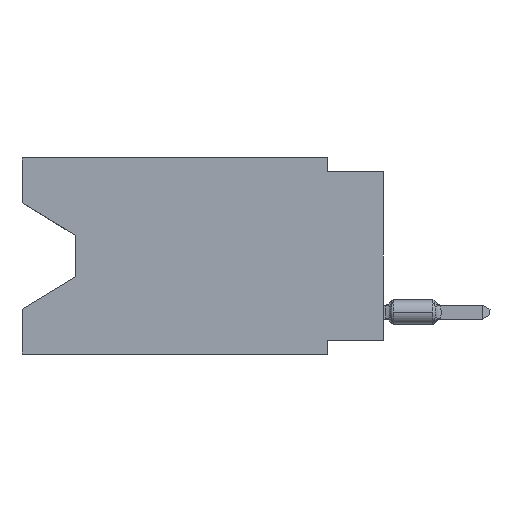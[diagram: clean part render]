
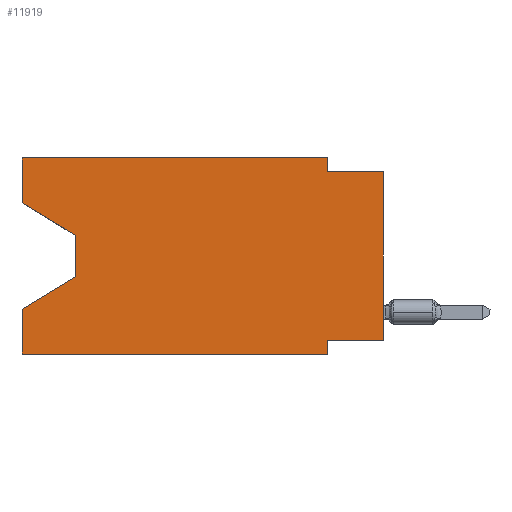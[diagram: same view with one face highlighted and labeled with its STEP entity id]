
A CAD part, left-side view. The second image highlights one B-rep face of the part: STEP entity #11919.
In plain terms, the highlighted planar face has unit normal (-1, 0, 0).
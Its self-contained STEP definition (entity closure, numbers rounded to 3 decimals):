
#265 = DIRECTION ( 'NONE',  ( 0., 0., 1. ) ) ;
#654 = ORIENTED_EDGE ( 'NONE', *, *, #4400, .F. ) ;
#823 = PLANE ( 'NONE',  #14181 ) ;
#1098 = EDGE_CURVE ( 'NONE', #6949, #5626, #3951, .T. ) ;
#1354 = CARTESIAN_POINT ( 'NONE',  ( 0., 2.54, -8.89 ) ) ;
#1677 = VERTEX_POINT ( 'NONE', #11141 ) ;
#1715 = VERTEX_POINT ( 'NONE', #12490 ) ;
#1744 = CARTESIAN_POINT ( 'NONE',  ( 0., 2.54, -8.255 ) ) ;
#1812 = ORIENTED_EDGE ( 'NONE', *, *, #13902, .F. ) ;
#1820 = DIRECTION ( 'NONE',  ( 0., 0., -1. ) ) ;
#2035 = CARTESIAN_POINT ( 'NONE',  ( 0., 16.383, 0. ) ) ;
#2098 = VECTOR ( 'NONE', #13037, 1000. ) ;
#2214 = VERTEX_POINT ( 'NONE', #4270 ) ;
#2402 = CARTESIAN_POINT ( 'NONE',  ( 0., 16.383, -8.89 ) ) ;
#2649 = CARTESIAN_POINT ( 'NONE',  ( 0., 13.97, -5.385 ) ) ;
#2692 = EDGE_CURVE ( 'NONE', #5484, #7489, #3575, .T. ) ;
#2698 = DIRECTION ( 'NONE',  ( 0., -1., 0. ) ) ;
#2728 = DIRECTION ( 'NONE',  ( 0., 0., -1. ) ) ;
#2739 = VERTEX_POINT ( 'NONE', #2649 ) ;
#2799 = EDGE_CURVE ( 'NONE', #1677, #6949, #7518, .T. ) ;
#2878 = ORIENTED_EDGE ( 'NONE', *, *, #2692, .F. ) ;
#2987 = CARTESIAN_POINT ( 'NONE',  ( 0., 0., -0.635 ) ) ;
#3268 = EDGE_CURVE ( 'NONE', #1715, #4939, #3776, .T. ) ;
#3575 = LINE ( 'NONE', #5774, #4999 ) ;
#3587 = VECTOR ( 'NONE', #6198, 1000. ) ;
#3776 = LINE ( 'NONE', #8427, #2098 ) ;
#3791 = VECTOR ( 'NONE', #4378, 1000. ) ;
#3951 = LINE ( 'NONE', #10875, #9055 ) ;
#3972 = LINE ( 'NONE', #7248, #12291 ) ;
#4261 = VERTEX_POINT ( 'NONE', #2402 ) ;
#4266 = VECTOR ( 'NONE', #12143, 1000. ) ;
#4270 = CARTESIAN_POINT ( 'NONE',  ( 0., 13.97, -3.505 ) ) ;
#4378 = DIRECTION ( 'NONE',  ( 0., 0.855, -0.519 ) ) ;
#4400 = EDGE_CURVE ( 'NONE', #4261, #10344, #7506, .T. ) ;
#4460 = EDGE_CURVE ( 'NONE', #4261, #5626, #14266, .T. ) ;
#4526 = CARTESIAN_POINT ( 'NONE',  ( 0., 0., 0. ) ) ;
#4890 = DIRECTION ( 'NONE',  ( 0., 0., 1. ) ) ;
#4939 = VERTEX_POINT ( 'NONE', #2987 ) ;
#4984 = LINE ( 'NONE', #10981, #3587 ) ;
#4999 = VECTOR ( 'NONE', #8222, 1000. ) ;
#5248 = EDGE_CURVE ( 'NONE', #2214, #2739, #11901, .T. ) ;
#5326 = EDGE_LOOP ( 'NONE', ( #6303, #9908, #8295, #654, #8242, #13004, #9715, #8193, #8932, #6922, #2878, #1812 ) ) ;
#5356 = DIRECTION ( 'NONE',  ( 0., 0., -1. ) ) ;
#5474 = VECTOR ( 'NONE', #14259, 1000. ) ;
#5484 = VERTEX_POINT ( 'NONE', #7831 ) ;
#5626 = VERTEX_POINT ( 'NONE', #1354 ) ;
#5751 = VECTOR ( 'NONE', #5356, 1000. ) ;
#5774 = CARTESIAN_POINT ( 'NONE',  ( 0., 16.383, 0. ) ) ;
#5979 = VECTOR ( 'NONE', #2698, 1000. ) ;
#6056 = EDGE_CURVE ( 'NONE', #7489, #1715, #8346, .T. ) ;
#6198 = DIRECTION ( 'NONE',  ( 0., -0.855, -0.519 ) ) ;
#6269 = EDGE_CURVE ( 'NONE', #1677, #4939, #11215, .T. ) ;
#6303 = ORIENTED_EDGE ( 'NONE', *, *, #10984, .T. ) ;
#6466 = VECTOR ( 'NONE', #265, 1000. ) ;
#6922 = ORIENTED_EDGE ( 'NONE', *, *, #6056, .F. ) ;
#6949 = VERTEX_POINT ( 'NONE', #1744 ) ;
#7248 = CARTESIAN_POINT ( 'NONE',  ( 0., 16.383, 0. ) ) ;
#7489 = VERTEX_POINT ( 'NONE', #11447 ) ;
#7506 = LINE ( 'NONE', #12131, #6466 ) ;
#7518 = LINE ( 'NONE', #10934, #4266 ) ;
#7579 = CARTESIAN_POINT ( 'NONE',  ( 0., 16.383, -2.038 ) ) ;
#7831 = CARTESIAN_POINT ( 'NONE',  ( 0., 16.383, 0. ) ) ;
#7879 = CARTESIAN_POINT ( 'NONE',  ( 0., 13.97, -5.385 ) ) ;
#8193 = ORIENTED_EDGE ( 'NONE', *, *, #6269, .T. ) ;
#8201 = VECTOR ( 'NONE', #12417, 1000. ) ;
#8222 = DIRECTION ( 'NONE',  ( 0., -1., 0. ) ) ;
#8242 = ORIENTED_EDGE ( 'NONE', *, *, #4460, .T. ) ;
#8295 = ORIENTED_EDGE ( 'NONE', *, *, #13308, .T. ) ;
#8346 = LINE ( 'NONE', #9556, #5751 ) ;
#8427 = CARTESIAN_POINT ( 'NONE',  ( 0., 0., -0.635 ) ) ;
#8501 = CARTESIAN_POINT ( 'NONE',  ( 0., 16.383, -8.89 ) ) ;
#8932 = ORIENTED_EDGE ( 'NONE', *, *, #3268, .F. ) ;
#9055 = VECTOR ( 'NONE', #2728, 1000. ) ;
#9556 = CARTESIAN_POINT ( 'NONE',  ( 0., 2.54, 0. ) ) ;
#9715 = ORIENTED_EDGE ( 'NONE', *, *, #2799, .F. ) ;
#9908 = ORIENTED_EDGE ( 'NONE', *, *, #5248, .T. ) ;
#10237 = LINE ( 'NONE', #7879, #3791 ) ;
#10344 = VERTEX_POINT ( 'NONE', #12467 ) ;
#10843 = CARTESIAN_POINT ( 'NONE',  ( 0., 13.97, -3.505 ) ) ;
#10875 = CARTESIAN_POINT ( 'NONE',  ( 0., 2.54, -8.89 ) ) ;
#10934 = CARTESIAN_POINT ( 'NONE',  ( 0., 0., -8.255 ) ) ;
#10981 = CARTESIAN_POINT ( 'NONE',  ( 0., 16.383, -2.038 ) ) ;
#10984 = EDGE_CURVE ( 'NONE', #13200, #2214, #4984, .T. ) ;
#11141 = CARTESIAN_POINT ( 'NONE',  ( 0., 0., -8.255 ) ) ;
#11215 = LINE ( 'NONE', #4526, #8201 ) ;
#11332 = DIRECTION ( 'NONE',  ( 1., 0., 0. ) ) ;
#11447 = CARTESIAN_POINT ( 'NONE',  ( 0., 2.54, 0. ) ) ;
#11901 = LINE ( 'NONE', #10843, #5474 ) ;
#11919 = ADVANCED_FACE ( 'NONE', ( #12231 ), #823, .F. ) ;
#12131 = CARTESIAN_POINT ( 'NONE',  ( 0., 16.383, 0. ) ) ;
#12143 = DIRECTION ( 'NONE',  ( 0., 1., 0. ) ) ;
#12231 = FACE_OUTER_BOUND ( 'NONE', #5326, .T. ) ;
#12291 = VECTOR ( 'NONE', #4890, 1000. ) ;
#12417 = DIRECTION ( 'NONE',  ( 0., 0., 1. ) ) ;
#12467 = CARTESIAN_POINT ( 'NONE',  ( 0., 16.383, -6.852 ) ) ;
#12490 = CARTESIAN_POINT ( 'NONE',  ( 0., 2.54, -0.635 ) ) ;
#13004 = ORIENTED_EDGE ( 'NONE', *, *, #1098, .F. ) ;
#13037 = DIRECTION ( 'NONE',  ( 0., -1., 0. ) ) ;
#13200 = VERTEX_POINT ( 'NONE', #7579 ) ;
#13308 = EDGE_CURVE ( 'NONE', #2739, #10344, #10237, .T. ) ;
#13902 = EDGE_CURVE ( 'NONE', #13200, #5484, #3972, .T. ) ;
#14181 = AXIS2_PLACEMENT_3D ( 'NONE', #2035, #11332, #1820 ) ;
#14259 = DIRECTION ( 'NONE',  ( 0., 0., -1. ) ) ;
#14266 = LINE ( 'NONE', #8501, #5979 ) ;
